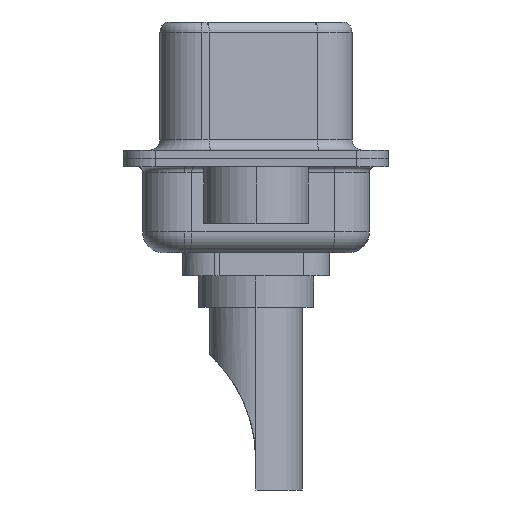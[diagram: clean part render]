
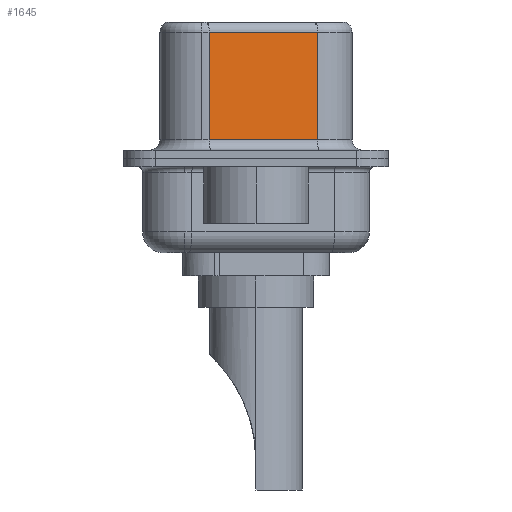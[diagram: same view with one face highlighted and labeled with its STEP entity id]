
A CAD part, left-side view. The second image highlights one B-rep face of the part: STEP entity #1645.
In plain terms, the highlighted planar face has unit normal (-0.985, -0.174, 0).
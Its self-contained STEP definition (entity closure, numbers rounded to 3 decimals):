
#1204 = LINE ( 'NONE', #20742, #18613 ) ;
#1645 = ADVANCED_FACE ( 'NONE', ( #2298 ), #17457, .F. ) ;
#1915 = VERTEX_POINT ( 'NONE', #6491 ) ;
#2298 = FACE_OUTER_BOUND ( 'NONE', #13222, .T. ) ;
#2347 = LINE ( 'NONE', #16023, #15224 ) ;
#3487 = DIRECTION ( 'NONE',  ( 0., 0., -1. ) ) ;
#3613 = EDGE_CURVE ( 'NONE', #7865, #13050, #5690, .T. ) ;
#5652 = ORIENTED_EDGE ( 'NONE', *, *, #20902, .T. ) ;
#5690 = LINE ( 'NONE', #7346, #6195 ) ;
#5739 = ORIENTED_EDGE ( 'NONE', *, *, #9719, .T. ) ;
#6195 = VECTOR ( 'NONE', #3487, 1000. ) ;
#6491 = CARTESIAN_POINT ( 'NONE',  ( 3.67, 2.233, 6.02 ) ) ;
#7346 = CARTESIAN_POINT ( 'NONE',  ( 4.58, -2.927, 6.52 ) ) ;
#7865 = VERTEX_POINT ( 'NONE', #20660 ) ;
#8944 = LINE ( 'NONE', #12157, #17350 ) ;
#9088 = CARTESIAN_POINT ( 'NONE',  ( 4.58, -2.927, 6.52 ) ) ;
#9122 = CARTESIAN_POINT ( 'NONE',  ( 4.58, -2.927, 0.9 ) ) ;
#9285 = DIRECTION ( 'NONE',  ( -0.174, 0.985, 0. ) ) ;
#9719 = EDGE_CURVE ( 'NONE', #1915, #20188, #8944, .T. ) ;
#10974 = CARTESIAN_POINT ( 'NONE',  ( 3.67, 2.233, 0.9 ) ) ;
#11505 = EDGE_CURVE ( 'NONE', #20188, #13050, #1204, .T. ) ;
#12157 = CARTESIAN_POINT ( 'NONE',  ( 3.67, 2.233, 6.52 ) ) ;
#13050 = VERTEX_POINT ( 'NONE', #9122 ) ;
#13222 = EDGE_LOOP ( 'NONE', ( #15571, #5652, #5739, #21781 ) ) ;
#13319 = DIRECTION ( 'NONE',  ( -0.174, 0.985, 0. ) ) ;
#15224 = VECTOR ( 'NONE', #9285, 1000. ) ;
#15571 = ORIENTED_EDGE ( 'NONE', *, *, #3613, .F. ) ;
#16023 = CARTESIAN_POINT ( 'NONE',  ( 4.58, -2.927, 6.02 ) ) ;
#16932 = DIRECTION ( 'NONE',  ( 0.174, -0.985, 0. ) ) ;
#17350 = VECTOR ( 'NONE', #21536, 1000. ) ;
#17457 = PLANE ( 'NONE',  #20548 ) ;
#18613 = VECTOR ( 'NONE', #16932, 1000. ) ;
#19848 = DIRECTION ( 'NONE',  ( 0.985, 0.174, 0. ) ) ;
#20188 = VERTEX_POINT ( 'NONE', #10974 ) ;
#20548 = AXIS2_PLACEMENT_3D ( 'NONE', #9088, #19848, #13319 ) ;
#20660 = CARTESIAN_POINT ( 'NONE',  ( 4.58, -2.927, 6.02 ) ) ;
#20742 = CARTESIAN_POINT ( 'NONE',  ( 4.58, -2.927, 0.9 ) ) ;
#20902 = EDGE_CURVE ( 'NONE', #7865, #1915, #2347, .T. ) ;
#21536 = DIRECTION ( 'NONE',  ( 0., 0., -1. ) ) ;
#21781 = ORIENTED_EDGE ( 'NONE', *, *, #11505, .T. ) ;
